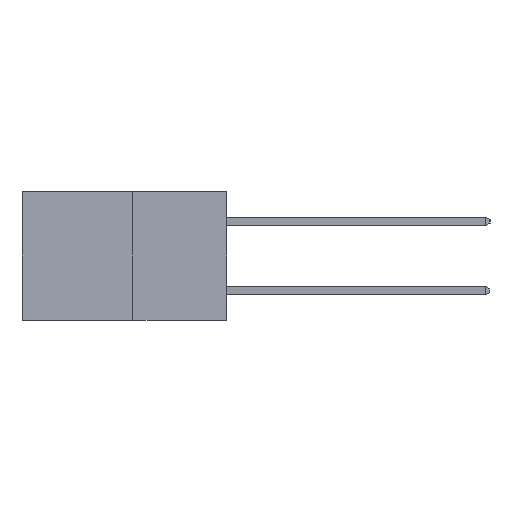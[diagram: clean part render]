
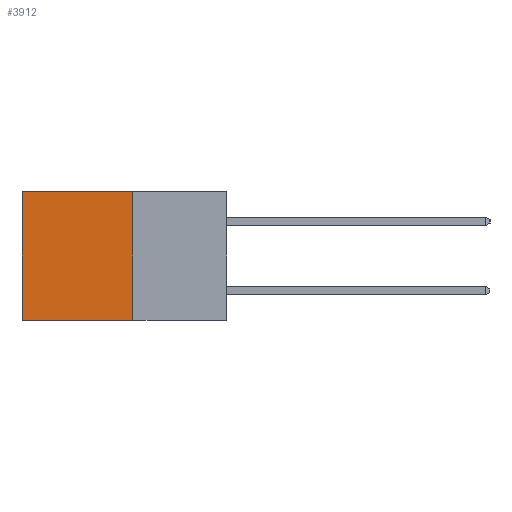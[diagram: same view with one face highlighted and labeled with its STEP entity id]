
A CAD part, left-side view. The second image highlights one B-rep face of the part: STEP entity #3912.
In plain terms, the highlighted planar face has unit normal (-1, 0, 0).
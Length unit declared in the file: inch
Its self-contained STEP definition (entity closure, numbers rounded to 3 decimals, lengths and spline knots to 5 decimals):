
#486 = DIRECTION ( 'NONE',  ( 1., 0., 0. ) ) ;
#1300 = DIRECTION ( 'NONE',  ( 0., 1., 0. ) ) ;
#1535 = FACE_OUTER_BOUND ( 'NONE', #15045, .T. ) ;
#2187 = VERTEX_POINT ( 'NONE', #2496 ) ;
#2428 = DIRECTION ( 'NONE',  ( 0., 1., 0. ) ) ;
#2440 = VECTOR ( 'NONE', #14827, 39.37008 ) ;
#2496 = CARTESIAN_POINT ( 'NONE',  ( 0.277, 0.59, -0.37 ) ) ;
#3401 = CARTESIAN_POINT ( 'NONE',  ( 0.277, 0.27, -0.37 ) ) ;
#3912 = ADVANCED_FACE ( 'NONE', ( #1535 ), #6865, .F. ) ;
#4085 = AXIS2_PLACEMENT_3D ( 'NONE', #6959, #486, #4098 ) ;
#4098 = DIRECTION ( 'NONE',  ( 0., 0., -1. ) ) ;
#4559 = VERTEX_POINT ( 'NONE', #5980 ) ;
#5310 = CARTESIAN_POINT ( 'NONE',  ( 0.277, 0.27, -0.37 ) ) ;
#5566 = LINE ( 'NONE', #13588, #11520 ) ;
#5980 = CARTESIAN_POINT ( 'NONE',  ( 0.277, 0.27, 0. ) ) ;
#6346 = LINE ( 'NONE', #8099, #2440 ) ;
#6865 = PLANE ( 'NONE',  #4085 ) ;
#6959 = CARTESIAN_POINT ( 'NONE',  ( 0.277, 0.27, -0.37 ) ) ;
#7599 = VERTEX_POINT ( 'NONE', #5310 ) ;
#7720 = EDGE_CURVE ( 'NONE', #7599, #2187, #14641, .T. ) ;
#8099 = CARTESIAN_POINT ( 'NONE',  ( 0.277, 0.27, -0.37 ) ) ;
#8900 = EDGE_CURVE ( 'NONE', #4559, #7599, #6346, .T. ) ;
#9543 = ORIENTED_EDGE ( 'NONE', *, *, #11920, .T. ) ;
#9626 = ORIENTED_EDGE ( 'NONE', *, *, #7720, .F. ) ;
#9724 = ORIENTED_EDGE ( 'NONE', *, *, #8900, .F. ) ;
#9832 = ORIENTED_EDGE ( 'NONE', *, *, #13037, .T. ) ;
#10988 = CARTESIAN_POINT ( 'NONE',  ( 0.277, 0.59, 0. ) ) ;
#11520 = VECTOR ( 'NONE', #14671, 39.37008 ) ;
#11590 = VERTEX_POINT ( 'NONE', #10988 ) ;
#11794 = VECTOR ( 'NONE', #2428, 39.37008 ) ;
#11920 = EDGE_CURVE ( 'NONE', #11590, #2187, #5566, .T. ) ;
#13037 = EDGE_CURVE ( 'NONE', #4559, #11590, #13676, .T. ) ;
#13092 = CARTESIAN_POINT ( 'NONE',  ( 0.277, 0.27, 0. ) ) ;
#13338 = VECTOR ( 'NONE', #1300, 39.37008 ) ;
#13588 = CARTESIAN_POINT ( 'NONE',  ( 0.277, 0.59, -0.37 ) ) ;
#13676 = LINE ( 'NONE', #13092, #13338 ) ;
#14641 = LINE ( 'NONE', #3401, #11794 ) ;
#14671 = DIRECTION ( 'NONE',  ( 0., 0., -1. ) ) ;
#14827 = DIRECTION ( 'NONE',  ( 0., 0., -1. ) ) ;
#15045 = EDGE_LOOP ( 'NONE', ( #9543, #9626, #9724, #9832 ) ) ;
